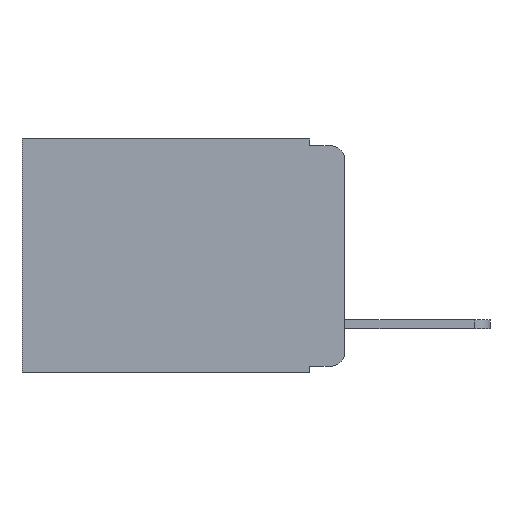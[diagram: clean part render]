
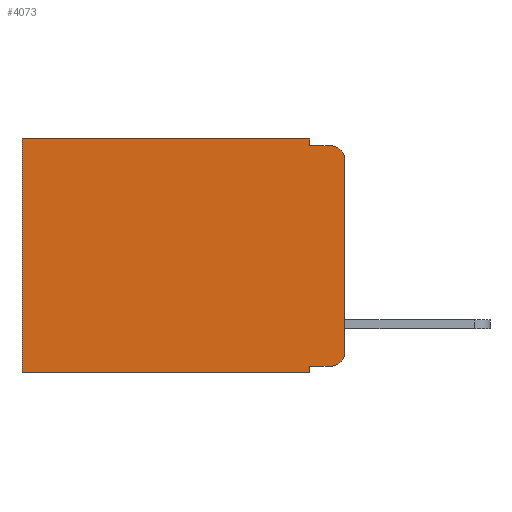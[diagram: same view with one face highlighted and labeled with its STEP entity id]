
A CAD part, left-side view. The second image highlights one B-rep face of the part: STEP entity #4073.
In plain terms, the highlighted planar face has unit normal (-1, 0, 0).
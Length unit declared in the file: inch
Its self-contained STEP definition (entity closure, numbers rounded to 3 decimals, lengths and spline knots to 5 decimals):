
#384 = LINE ( 'NONE', #11376, #12764 ) ;
#577 = VERTEX_POINT ( 'NONE', #10777 ) ;
#1184 = LINE ( 'NONE', #10195, #9330 ) ;
#1402 = CARTESIAN_POINT ( 'NONE',  ( 0.298, 0.051, 0. ) ) ;
#1436 = CARTESIAN_POINT ( 'NONE',  ( 0.298, 0.051, -0.333 ) ) ;
#1807 = CARTESIAN_POINT ( 'NONE',  ( 0.298, 0., -0.313 ) ) ;
#2133 = VECTOR ( 'NONE', #7935, 39.37008 ) ;
#2250 = FACE_OUTER_BOUND ( 'NONE', #6441, .T. ) ;
#2469 = LINE ( 'NONE', #6038, #2133 ) ;
#3160 = LINE ( 'NONE', #1402, #5386 ) ;
#3383 = VECTOR ( 'NONE', #4658, 39.37008 ) ;
#3406 = DIRECTION ( 'NONE',  ( 0., 0., -1. ) ) ;
#3425 = DIRECTION ( 'NONE',  ( 1., 0., 0. ) ) ;
#3582 = VERTEX_POINT ( 'NONE', #11873 ) ;
#4073 = ADVANCED_FACE ( 'NONE', ( #2250 ), #11117, .F. ) ;
#4092 = CARTESIAN_POINT ( 'NONE',  ( 0.298, 0.02, -0.313 ) ) ;
#4395 = VERTEX_POINT ( 'NONE', #7726 ) ;
#4487 = VERTEX_POINT ( 'NONE', #8024 ) ;
#4508 = VERTEX_POINT ( 'NONE', #8090 ) ;
#4602 = ORIENTED_EDGE ( 'NONE', *, *, #9822, .F. ) ;
#4658 = DIRECTION ( 'NONE',  ( 0., -1., 0. ) ) ;
#4732 = ORIENTED_EDGE ( 'NONE', *, *, #10397, .T. ) ;
#4810 = ORIENTED_EDGE ( 'NONE', *, *, #9457, .F. ) ;
#5019 = ORIENTED_EDGE ( 'NONE', *, *, #8888, .F. ) ;
#5104 = LINE ( 'NONE', #12399, #7566 ) ;
#5137 = DIRECTION ( 'NONE',  ( 0., 0., -1. ) ) ;
#5147 = AXIS2_PLACEMENT_3D ( 'NONE', #9253, #3425, #3406 ) ;
#5202 = ORIENTED_EDGE ( 'NONE', *, *, #8300, .T. ) ;
#5205 = ORIENTED_EDGE ( 'NONE', *, *, #8769, .T. ) ;
#5386 = VECTOR ( 'NONE', #12052, 39.37008 ) ;
#5493 = DIRECTION ( 'NONE',  ( 0., 1., 0. ) ) ;
#5556 = ORIENTED_EDGE ( 'NONE', *, *, #9327, .F. ) ;
#5583 = ORIENTED_EDGE ( 'NONE', *, *, #12594, .F. ) ;
#5733 = ORIENTED_EDGE ( 'NONE', *, *, #8233, .T. ) ;
#5784 = ORIENTED_EDGE ( 'NONE', *, *, #6811, .T. ) ;
#5886 = DIRECTION ( 'NONE',  ( 0., -1., 0. ) ) ;
#5960 = CARTESIAN_POINT ( 'NONE',  ( 0.298, 0.02, -0.03 ) ) ;
#6038 = CARTESIAN_POINT ( 'NONE',  ( 0.298, 0., 0. ) ) ;
#6256 = CIRCLE ( 'NONE', #8302, 0.02 ) ;
#6435 = DIRECTION ( 'NONE',  ( 0., 0., -1. ) ) ;
#6441 = EDGE_LOOP ( 'NONE', ( #4602, #4732, #4810, #5019, #5202, #5205, #5556, #5583, #5733, #5784 ) ) ;
#6537 = VECTOR ( 'NONE', #5886, 39.37008 ) ;
#6811 = EDGE_CURVE ( 'NONE', #4487, #9816, #6256, .T. ) ;
#6917 = CARTESIAN_POINT ( 'NONE',  ( 0.298, 0.051, 0. ) ) ;
#6945 = DIRECTION ( 'NONE',  ( 0., 0., -1. ) ) ;
#7028 = VECTOR ( 'NONE', #5493, 39.37008 ) ;
#7085 = DIRECTION ( 'NONE',  ( 0., 0., -1. ) ) ;
#7566 = VECTOR ( 'NONE', #7085, 39.37008 ) ;
#7719 = VERTEX_POINT ( 'NONE', #7951 ) ;
#7726 = CARTESIAN_POINT ( 'NONE',  ( 0.298, 0.473, -0.343 ) ) ;
#7935 = DIRECTION ( 'NONE',  ( 0., 1., 0. ) ) ;
#7951 = CARTESIAN_POINT ( 'NONE',  ( 0.298, 0.02, -0.01 ) ) ;
#8024 = CARTESIAN_POINT ( 'NONE',  ( 0.298, 0.02, -0.333 ) ) ;
#8034 = CARTESIAN_POINT ( 'NONE',  ( 0.298, 0.051, -0.343 ) ) ;
#8090 = CARTESIAN_POINT ( 'NONE',  ( 0.298, 0., -0.03 ) ) ;
#8233 = EDGE_CURVE ( 'NONE', #10286, #4487, #9074, .T. ) ;
#8300 = EDGE_CURVE ( 'NONE', #12621, #577, #2469, .T. ) ;
#8302 = AXIS2_PLACEMENT_3D ( 'NONE', #4092, #10630, #5137 ) ;
#8358 = VERTEX_POINT ( 'NONE', #8034 ) ;
#8769 = EDGE_CURVE ( 'NONE', #577, #4395, #1184, .T. ) ;
#8888 = EDGE_CURVE ( 'NONE', #12621, #3582, #3160, .T. ) ;
#9074 = LINE ( 'NONE', #12201, #6537 ) ;
#9253 = CARTESIAN_POINT ( 'NONE',  ( 0.298, 0., 0. ) ) ;
#9327 = EDGE_CURVE ( 'NONE', #8358, #4395, #12133, .T. ) ;
#9330 = VECTOR ( 'NONE', #6435, 39.37008 ) ;
#9457 = EDGE_CURVE ( 'NONE', #3582, #7719, #10963, .T. ) ;
#9816 = VERTEX_POINT ( 'NONE', #1807 ) ;
#9822 = EDGE_CURVE ( 'NONE', #4508, #9816, #5104, .T. ) ;
#10195 = CARTESIAN_POINT ( 'NONE',  ( 0.298, 0.473, 0. ) ) ;
#10224 = CARTESIAN_POINT ( 'NONE',  ( 0.298, 0.051, -0.01 ) ) ;
#10286 = VERTEX_POINT ( 'NONE', #1436 ) ;
#10397 = EDGE_CURVE ( 'NONE', #4508, #7719, #12543, .T. ) ;
#10630 = DIRECTION ( 'NONE',  ( -1., 0., 0. ) ) ;
#10777 = CARTESIAN_POINT ( 'NONE',  ( 0.298, 0.473, 0. ) ) ;
#10949 = CARTESIAN_POINT ( 'NONE',  ( 0.298, 0., -0.343 ) ) ;
#10963 = LINE ( 'NONE', #10224, #3383 ) ;
#11117 = PLANE ( 'NONE',  #5147 ) ;
#11376 = CARTESIAN_POINT ( 'NONE',  ( 0.298, 0.051, 0. ) ) ;
#11382 = AXIS2_PLACEMENT_3D ( 'NONE', #5960, #12278, #6945 ) ;
#11873 = CARTESIAN_POINT ( 'NONE',  ( 0.298, 0.051, -0.01 ) ) ;
#12052 = DIRECTION ( 'NONE',  ( 0., 0., -1. ) ) ;
#12133 = LINE ( 'NONE', #10949, #7028 ) ;
#12201 = CARTESIAN_POINT ( 'NONE',  ( 0.298, 0.051, -0.333 ) ) ;
#12204 = DIRECTION ( 'NONE',  ( 0., 0., -1. ) ) ;
#12278 = DIRECTION ( 'NONE',  ( -1., 0., 0. ) ) ;
#12399 = CARTESIAN_POINT ( 'NONE',  ( 0.298, 0., 0. ) ) ;
#12543 = CIRCLE ( 'NONE', #11382, 0.02 ) ;
#12594 = EDGE_CURVE ( 'NONE', #10286, #8358, #384, .T. ) ;
#12621 = VERTEX_POINT ( 'NONE', #6917 ) ;
#12764 = VECTOR ( 'NONE', #12204, 39.37008 ) ;
